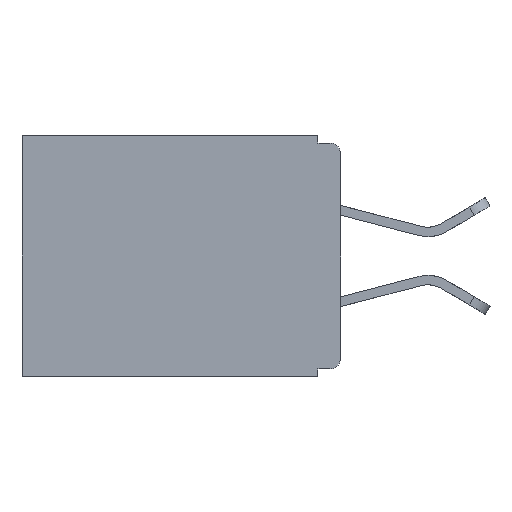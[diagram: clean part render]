
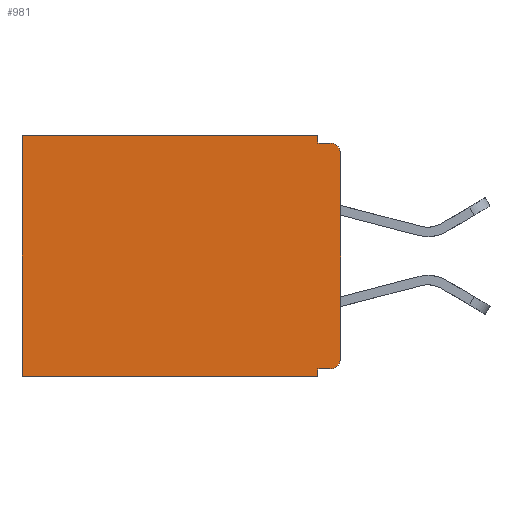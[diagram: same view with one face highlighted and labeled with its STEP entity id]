
A CAD part, left-side view. The second image highlights one B-rep face of the part: STEP entity #981.
In plain terms, the highlighted planar face has unit normal (-1, 0, 0).
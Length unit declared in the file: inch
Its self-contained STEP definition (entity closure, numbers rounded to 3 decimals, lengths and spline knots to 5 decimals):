
#129 = VECTOR ( 'NONE', #12975, 39.37008 ) ;
#206 = ORIENTED_EDGE ( 'NONE', *, *, #10616, .F. ) ;
#324 = ORIENTED_EDGE ( 'NONE', *, *, #7878, .F. ) ;
#430 = AXIS2_PLACEMENT_3D ( 'NONE', #5748, #10740, #10356 ) ;
#473 = VERTEX_POINT ( 'NONE', #9874 ) ;
#554 = ORIENTED_EDGE ( 'NONE', *, *, #2434, .T. ) ;
#759 = LINE ( 'NONE', #4313, #8707 ) ;
#870 = LINE ( 'NONE', #13324, #3423 ) ;
#937 = LINE ( 'NONE', #5925, #6221 ) ;
#981 = ADVANCED_FACE ( 'NONE', ( #6163 ), #9955, .F. ) ;
#1063 = DIRECTION ( 'NONE',  ( 0., -1., 0. ) ) ;
#1071 = VERTEX_POINT ( 'NONE', #13065 ) ;
#1320 = ORIENTED_EDGE ( 'NONE', *, *, #8947, .T. ) ;
#1526 = ORIENTED_EDGE ( 'NONE', *, *, #12732, .T. ) ;
#1628 = ORIENTED_EDGE ( 'NONE', *, *, #3889, .F. ) ;
#1929 = CARTESIAN_POINT ( 'NONE',  ( 0.3, 0., -0.305 ) ) ;
#2368 = VERTEX_POINT ( 'NONE', #2751 ) ;
#2434 = EDGE_CURVE ( 'NONE', #11711, #3702, #2526, .T. ) ;
#2526 = CIRCLE ( 'NONE', #11795, 0.015 ) ;
#2641 = VECTOR ( 'NONE', #7118, 39.37008 ) ;
#2649 = CARTESIAN_POINT ( 'NONE',  ( 0.3, 0.437, -0.33 ) ) ;
#2700 = DIRECTION ( 'NONE',  ( -1., 0., 0. ) ) ;
#2751 = CARTESIAN_POINT ( 'NONE',  ( 0.3, 0.031, -0.33 ) ) ;
#2979 = LINE ( 'NONE', #12995, #129 ) ;
#2995 = VECTOR ( 'NONE', #8797, 39.37008 ) ;
#3062 = ORIENTED_EDGE ( 'NONE', *, *, #7441, .F. ) ;
#3423 = VECTOR ( 'NONE', #1063, 39.37008 ) ;
#3605 = VERTEX_POINT ( 'NONE', #3797 ) ;
#3702 = VERTEX_POINT ( 'NONE', #1929 ) ;
#3797 = CARTESIAN_POINT ( 'NONE',  ( 0.3, 0.437, 0. ) ) ;
#3889 = EDGE_CURVE ( 'NONE', #2368, #1071, #9372, .T. ) ;
#4027 = VECTOR ( 'NONE', #12767, 39.37008 ) ;
#4108 = CARTESIAN_POINT ( 'NONE',  ( 0.3, 0.015, -0.32 ) ) ;
#4313 = CARTESIAN_POINT ( 'NONE',  ( 0.3, 0., -0.33 ) ) ;
#4326 = DIRECTION ( 'NONE',  ( 0., 0., -1. ) ) ;
#4363 = CARTESIAN_POINT ( 'NONE',  ( 0.3, 0.031, 0. ) ) ;
#4447 = VERTEX_POINT ( 'NONE', #11572 ) ;
#5748 = CARTESIAN_POINT ( 'NONE',  ( 0.3, 0., -0.33 ) ) ;
#5883 = DIRECTION ( 'NONE',  ( 0., 1., 0. ) ) ;
#5925 = CARTESIAN_POINT ( 'NONE',  ( 0.3, 0., 0. ) ) ;
#6163 = FACE_OUTER_BOUND ( 'NONE', #8662, .T. ) ;
#6221 = VECTOR ( 'NONE', #5883, 39.37008 ) ;
#6683 = ORIENTED_EDGE ( 'NONE', *, *, #9193, .F. ) ;
#6732 = CARTESIAN_POINT ( 'NONE',  ( 0.3, 0., -0.32 ) ) ;
#7118 = DIRECTION ( 'NONE',  ( 0., 1., 0. ) ) ;
#7441 = EDGE_CURVE ( 'NONE', #11711, #13337, #8132, .T. ) ;
#7878 = EDGE_CURVE ( 'NONE', #13337, #2368, #2979, .T. ) ;
#7895 = VERTEX_POINT ( 'NONE', #13181 ) ;
#7994 = VERTEX_POINT ( 'NONE', #12232 ) ;
#8132 = LINE ( 'NONE', #6732, #2641 ) ;
#8508 = ORIENTED_EDGE ( 'NONE', *, *, #12153, .T. ) ;
#8662 = EDGE_LOOP ( 'NONE', ( #6683, #8508, #11425, #206, #1320, #1526, #1628, #324, #3062, #554 ) ) ;
#8707 = VECTOR ( 'NONE', #4326, 39.37008 ) ;
#8754 = LINE ( 'NONE', #2649, #2995 ) ;
#8797 = DIRECTION ( 'NONE',  ( 0., 0., -1. ) ) ;
#8842 = CARTESIAN_POINT ( 'NONE',  ( 0.3, 0.015, -0.025 ) ) ;
#8947 = EDGE_CURVE ( 'NONE', #473, #3605, #937, .T. ) ;
#9193 = EDGE_CURVE ( 'NONE', #7895, #3702, #759, .T. ) ;
#9372 = LINE ( 'NONE', #9708, #4027 ) ;
#9708 = CARTESIAN_POINT ( 'NONE',  ( 0.3, 0., -0.33 ) ) ;
#9764 = CARTESIAN_POINT ( 'NONE',  ( 0.3, 0.031, -0.32 ) ) ;
#9826 = DIRECTION ( 'NONE',  ( 0., 0., -1. ) ) ;
#9874 = CARTESIAN_POINT ( 'NONE',  ( 0.3, 0.031, 0. ) ) ;
#9955 = PLANE ( 'NONE',  #430 ) ;
#10028 = VECTOR ( 'NONE', #11376, 39.37008 ) ;
#10306 = CIRCLE ( 'NONE', #11267, 0.015 ) ;
#10356 = DIRECTION ( 'NONE',  ( 0., 0., -1. ) ) ;
#10462 = DIRECTION ( 'NONE',  ( -1., 0., 0. ) ) ;
#10578 = DIRECTION ( 'NONE',  ( 0., 0., -1. ) ) ;
#10616 = EDGE_CURVE ( 'NONE', #473, #4447, #12754, .T. ) ;
#10722 = CARTESIAN_POINT ( 'NONE',  ( 0.3, 0.015, -0.305 ) ) ;
#10740 = DIRECTION ( 'NONE',  ( 1., 0., 0. ) ) ;
#11197 = EDGE_CURVE ( 'NONE', #4447, #7994, #870, .T. ) ;
#11267 = AXIS2_PLACEMENT_3D ( 'NONE', #8842, #2700, #9826 ) ;
#11376 = DIRECTION ( 'NONE',  ( 0., 0., -1. ) ) ;
#11425 = ORIENTED_EDGE ( 'NONE', *, *, #11197, .F. ) ;
#11572 = CARTESIAN_POINT ( 'NONE',  ( 0.3, 0.031, -0.01 ) ) ;
#11711 = VERTEX_POINT ( 'NONE', #4108 ) ;
#11795 = AXIS2_PLACEMENT_3D ( 'NONE', #10722, #10462, #10578 ) ;
#12153 = EDGE_CURVE ( 'NONE', #7895, #7994, #10306, .T. ) ;
#12232 = CARTESIAN_POINT ( 'NONE',  ( 0.3, 0.015, -0.01 ) ) ;
#12732 = EDGE_CURVE ( 'NONE', #3605, #1071, #8754, .T. ) ;
#12754 = LINE ( 'NONE', #4363, #10028 ) ;
#12767 = DIRECTION ( 'NONE',  ( 0., 1., 0. ) ) ;
#12975 = DIRECTION ( 'NONE',  ( 0., 0., -1. ) ) ;
#12995 = CARTESIAN_POINT ( 'NONE',  ( 0.3, 0.031, -0.33 ) ) ;
#13065 = CARTESIAN_POINT ( 'NONE',  ( 0.3, 0.437, -0.33 ) ) ;
#13181 = CARTESIAN_POINT ( 'NONE',  ( 0.3, 0., -0.025 ) ) ;
#13324 = CARTESIAN_POINT ( 'NONE',  ( 0.3, 0., -0.01 ) ) ;
#13337 = VERTEX_POINT ( 'NONE', #9764 ) ;
